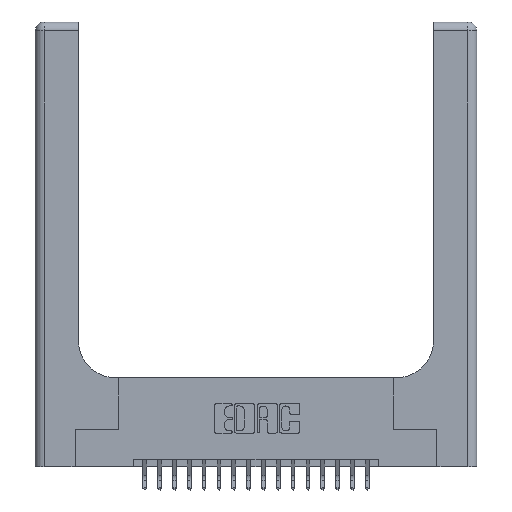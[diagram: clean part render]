
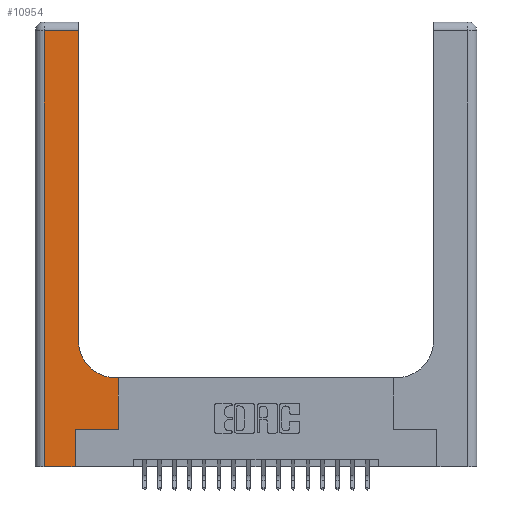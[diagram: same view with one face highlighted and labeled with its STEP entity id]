
A CAD part, top view. The second image highlights one B-rep face of the part: STEP entity #10954.
In plain terms, the highlighted planar face has unit normal (0, 0, 1).
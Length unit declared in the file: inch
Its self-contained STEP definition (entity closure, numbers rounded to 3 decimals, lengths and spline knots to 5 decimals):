
#34 = VERTEX_POINT ( 'NONE', #5143 ) ;
#359 = CARTESIAN_POINT ( 'NONE',  ( 0.269, 0., 0.37 ) ) ;
#1102 = CARTESIAN_POINT ( 'NONE',  ( 0.2915, 2.94, 0.37 ) ) ;
#1155 = VECTOR ( 'NONE', #4348, 39.37008 ) ;
#1278 = EDGE_CURVE ( 'NONE', #4203, #17108, #5117, .T. ) ;
#1385 = CARTESIAN_POINT ( 'NONE',  ( 0.2915, 0.6, 0.37 ) ) ;
#1469 = EDGE_CURVE ( 'NONE', #17108, #10490, #16774, .T. ) ;
#1769 = AXIS2_PLACEMENT_3D ( 'NONE', #1956, #6693, #11879 ) ;
#1956 = CARTESIAN_POINT ( 'NONE',  ( 0., 3., 0.37 ) ) ;
#2040 = ORIENTED_EDGE ( 'NONE', *, *, #9418, .T. ) ;
#2651 = ORIENTED_EDGE ( 'NONE', *, *, #3317, .T. ) ;
#2938 = DIRECTION ( 'NONE',  ( 1., 0., 0. ) ) ;
#3136 = DIRECTION ( 'NONE',  ( -1., 0., 0. ) ) ;
#3140 = CARTESIAN_POINT ( 'NONE',  ( 0.5415, 0.85, 0.37 ) ) ;
#3168 = VECTOR ( 'NONE', #16119, 39.37008 ) ;
#3317 = EDGE_CURVE ( 'NONE', #11944, #16553, #4526, .T. ) ;
#4099 = EDGE_CURVE ( 'NONE', #34, #17839, #19261, .T. ) ;
#4203 = VERTEX_POINT ( 'NONE', #1102 ) ;
#4239 = VECTOR ( 'NONE', #17023, 39.37008 ) ;
#4306 = VECTOR ( 'NONE', #6482, 39.37008 ) ;
#4348 = DIRECTION ( 'NONE',  ( -1., 0., 0. ) ) ;
#4405 = DIRECTION ( 'NONE',  ( 1., 0., 0. ) ) ;
#4526 = LINE ( 'NONE', #1385, #1155 ) ;
#4642 = CARTESIAN_POINT ( 'NONE',  ( 0.269, 0.25, 0.37 ) ) ;
#4954 = CARTESIAN_POINT ( 'NONE',  ( 0.5585, 0.25, 0.37 ) ) ;
#5076 = EDGE_CURVE ( 'NONE', #17839, #19813, #20499, .T. ) ;
#5117 = LINE ( 'NONE', #6194, #17049 ) ;
#5143 = CARTESIAN_POINT ( 'NONE',  ( 0.269, 0., 0.37 ) ) ;
#5376 = EDGE_CURVE ( 'NONE', #19813, #11944, #16346, .T. ) ;
#5709 = CARTESIAN_POINT ( 'NONE',  ( 0.06, 3., 0.37 ) ) ;
#6194 = CARTESIAN_POINT ( 'NONE',  ( 0., 2.94, 0.37 ) ) ;
#6372 = CARTESIAN_POINT ( 'NONE',  ( 0., 0., 0.37 ) ) ;
#6482 = DIRECTION ( 'NONE',  ( 0., 1., 0. ) ) ;
#6693 = DIRECTION ( 'NONE',  ( 0., 0., -1. ) ) ;
#6845 = PLANE ( 'NONE',  #1769 ) ;
#7303 = VECTOR ( 'NONE', #14577, 39.37008 ) ;
#7453 = LINE ( 'NONE', #12849, #4306 ) ;
#7845 = CARTESIAN_POINT ( 'NONE',  ( 0.5585, 0.25, 0.37 ) ) ;
#8304 = EDGE_CURVE ( 'NONE', #16553, #12530, #17463, .T. ) ;
#8743 = ORIENTED_EDGE ( 'NONE', *, *, #12600, .T. ) ;
#9415 = VECTOR ( 'NONE', #4405, 39.37008 ) ;
#9418 = EDGE_CURVE ( 'NONE', #10490, #34, #9911, .T. ) ;
#9635 = ORIENTED_EDGE ( 'NONE', *, *, #1469, .T. ) ;
#9865 = CARTESIAN_POINT ( 'NONE',  ( 0.5415, 0.6, 0.37 ) ) ;
#9911 = LINE ( 'NONE', #6372, #3168 ) ;
#10490 = VERTEX_POINT ( 'NONE', #19263 ) ;
#10954 = ADVANCED_FACE ( 'NONE', ( #11622 ), #6845, .F. ) ;
#11399 = DIRECTION ( 'NONE',  ( 0., 0., -1. ) ) ;
#11622 = FACE_OUTER_BOUND ( 'NONE', #14974, .T. ) ;
#11879 = DIRECTION ( 'NONE',  ( -1., 0., 0. ) ) ;
#11944 = VERTEX_POINT ( 'NONE', #17652 ) ;
#12388 = ORIENTED_EDGE ( 'NONE', *, *, #5076, .T. ) ;
#12530 = VERTEX_POINT ( 'NONE', #17708 ) ;
#12600 = EDGE_CURVE ( 'NONE', #12530, #4203, #7453, .T. ) ;
#12849 = CARTESIAN_POINT ( 'NONE',  ( 0.2915, 3., 0.37 ) ) ;
#14151 = CARTESIAN_POINT ( 'NONE',  ( 0.269, 0.25, 0.37 ) ) ;
#14577 = DIRECTION ( 'NONE',  ( 0., 1., 0. ) ) ;
#14881 = ORIENTED_EDGE ( 'NONE', *, *, #4099, .T. ) ;
#14974 = EDGE_LOOP ( 'NONE', ( #8743, #19288, #9635, #2040, #14881, #12388, #17671, #2651, #17750 ) ) ;
#15555 = DIRECTION ( 'NONE',  ( 0., -1., 0. ) ) ;
#16119 = DIRECTION ( 'NONE',  ( 1., 0., 0. ) ) ;
#16346 = LINE ( 'NONE', #7845, #7303 ) ;
#16553 = VERTEX_POINT ( 'NONE', #9865 ) ;
#16774 = LINE ( 'NONE', #5709, #18591 ) ;
#17023 = DIRECTION ( 'NONE',  ( 0., 1., 0. ) ) ;
#17049 = VECTOR ( 'NONE', #3136, 39.37008 ) ;
#17108 = VERTEX_POINT ( 'NONE', #17932 ) ;
#17463 = CIRCLE ( 'NONE', #20899, 0.25 ) ;
#17652 = CARTESIAN_POINT ( 'NONE',  ( 0.5585, 0.6, 0.37 ) ) ;
#17671 = ORIENTED_EDGE ( 'NONE', *, *, #5376, .T. ) ;
#17708 = CARTESIAN_POINT ( 'NONE',  ( 0.2915, 0.85, 0.37 ) ) ;
#17750 = ORIENTED_EDGE ( 'NONE', *, *, #8304, .T. ) ;
#17839 = VERTEX_POINT ( 'NONE', #4642 ) ;
#17932 = CARTESIAN_POINT ( 'NONE',  ( 0.06, 2.94, 0.37 ) ) ;
#18591 = VECTOR ( 'NONE', #15555, 39.37008 ) ;
#19261 = LINE ( 'NONE', #359, #4239 ) ;
#19263 = CARTESIAN_POINT ( 'NONE',  ( 0.06, 0., 0.37 ) ) ;
#19288 = ORIENTED_EDGE ( 'NONE', *, *, #1278, .T. ) ;
#19813 = VERTEX_POINT ( 'NONE', #4954 ) ;
#20499 = LINE ( 'NONE', #14151, #9415 ) ;
#20899 = AXIS2_PLACEMENT_3D ( 'NONE', #3140, #11399, #2938 ) ;
